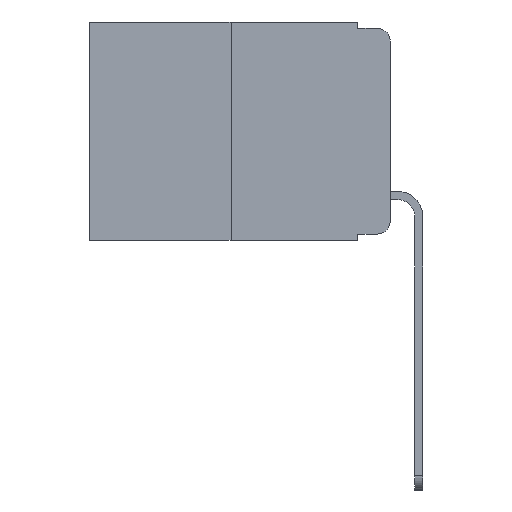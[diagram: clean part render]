
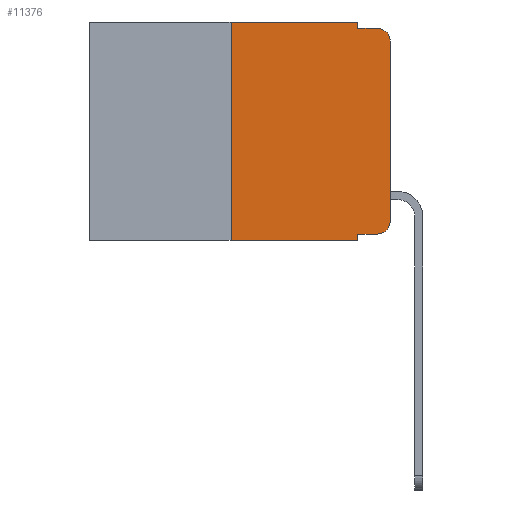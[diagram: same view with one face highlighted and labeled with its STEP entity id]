
A CAD part, left-side view. The second image highlights one B-rep face of the part: STEP entity #11376.
In plain terms, the highlighted planar face has unit normal (-1, 0, 0).
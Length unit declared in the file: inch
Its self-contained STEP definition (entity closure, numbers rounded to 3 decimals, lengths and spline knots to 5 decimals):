
#78 = VERTEX_POINT ( 'NONE', #9142 ) ;
#319 = VECTOR ( 'NONE', #1893, 39.37008 ) ;
#492 = LINE ( 'NONE', #1943, #319 ) ;
#668 = LINE ( 'NONE', #11216, #2247 ) ;
#675 = VECTOR ( 'NONE', #11264, 39.37008 ) ;
#968 = PLANE ( 'NONE',  #13444 ) ;
#1014 = DIRECTION ( 'NONE',  ( 1., 0., 0. ) ) ;
#1072 = DIRECTION ( 'NONE',  ( -1., 0., 0. ) ) ;
#1408 = VECTOR ( 'NONE', #3581, 39.37008 ) ;
#1508 = VECTOR ( 'NONE', #7893, 39.37008 ) ;
#1582 = EDGE_CURVE ( 'NONE', #3085, #9152, #4040, .T. ) ;
#1893 = DIRECTION ( 'NONE',  ( 0., -1., 0. ) ) ;
#1917 = AXIS2_PLACEMENT_3D ( 'NONE', #4322, #4279, #14426 ) ;
#1943 = CARTESIAN_POINT ( 'NONE',  ( 0., 0.051, -0.333 ) ) ;
#2247 = VECTOR ( 'NONE', #13514, 39.37008 ) ;
#2286 = ORIENTED_EDGE ( 'NONE', *, *, #2820, .F. ) ;
#2370 = CARTESIAN_POINT ( 'NONE',  ( 0., 0., 0. ) ) ;
#2820 = EDGE_CURVE ( 'NONE', #6180, #4557, #9934, .T. ) ;
#2931 = EDGE_CURVE ( 'NONE', #7066, #6180, #6783, .T. ) ;
#3085 = VERTEX_POINT ( 'NONE', #10618 ) ;
#3165 = CARTESIAN_POINT ( 'NONE',  ( 0., 0.051, -0.343 ) ) ;
#3506 = CARTESIAN_POINT ( 'NONE',  ( 0., 0.051, 0. ) ) ;
#3535 = CARTESIAN_POINT ( 'NONE',  ( 0., 0.051, -0.01 ) ) ;
#3581 = DIRECTION ( 'NONE',  ( 0., -1., 0. ) ) ;
#3651 = VERTEX_POINT ( 'NONE', #8904 ) ;
#3710 = EDGE_CURVE ( 'NONE', #7066, #8391, #3791, .T. ) ;
#3791 = LINE ( 'NONE', #4683, #1508 ) ;
#4040 = LINE ( 'NONE', #3535, #1408 ) ;
#4217 = ORIENTED_EDGE ( 'NONE', *, *, #2931, .F. ) ;
#4246 = LINE ( 'NONE', #3506, #10911 ) ;
#4269 = ORIENTED_EDGE ( 'NONE', *, *, #10042, .T. ) ;
#4279 = DIRECTION ( 'NONE',  ( -1., 0., 0. ) ) ;
#4322 = CARTESIAN_POINT ( 'NONE',  ( 0., 0.02, -0.03 ) ) ;
#4323 = CARTESIAN_POINT ( 'NONE',  ( 0., 0.051, 0. ) ) ;
#4557 = VERTEX_POINT ( 'NONE', #4323 ) ;
#4683 = CARTESIAN_POINT ( 'NONE',  ( 0., 0.473, -0.343 ) ) ;
#4719 = VECTOR ( 'NONE', #11214, 39.37008 ) ;
#5251 = CIRCLE ( 'NONE', #7163, 0.02 ) ;
#5389 = VERTEX_POINT ( 'NONE', #7640 ) ;
#5499 = DIRECTION ( 'NONE',  ( 0., 0., -1. ) ) ;
#5584 = CARTESIAN_POINT ( 'NONE',  ( 0., 0.25, 0. ) ) ;
#5716 = CIRCLE ( 'NONE', #1917, 0.02 ) ;
#5769 = LINE ( 'NONE', #2370, #4719 ) ;
#5912 = VECTOR ( 'NONE', #14518, 39.37008 ) ;
#6067 = EDGE_CURVE ( 'NONE', #5389, #3651, #5769, .T. ) ;
#6147 = ORIENTED_EDGE ( 'NONE', *, *, #6067, .T. ) ;
#6180 = VERTEX_POINT ( 'NONE', #13803 ) ;
#6581 = EDGE_CURVE ( 'NONE', #78, #5389, #5251, .T. ) ;
#6583 = CARTESIAN_POINT ( 'NONE',  ( 0., 0.473, 0. ) ) ;
#6783 = LINE ( 'NONE', #5584, #675 ) ;
#7066 = VERTEX_POINT ( 'NONE', #7863 ) ;
#7163 = AXIS2_PLACEMENT_3D ( 'NONE', #7831, #1072, #10055 ) ;
#7392 = ORIENTED_EDGE ( 'NONE', *, *, #6581, .T. ) ;
#7640 = CARTESIAN_POINT ( 'NONE',  ( 0., 0., -0.313 ) ) ;
#7831 = CARTESIAN_POINT ( 'NONE',  ( 0., 0.02, -0.313 ) ) ;
#7863 = CARTESIAN_POINT ( 'NONE',  ( 0., 0.25, -0.343 ) ) ;
#7893 = DIRECTION ( 'NONE',  ( 0., -1., 0. ) ) ;
#7967 = ORIENTED_EDGE ( 'NONE', *, *, #11808, .T. ) ;
#8049 = CARTESIAN_POINT ( 'NONE',  ( 0., 0.02, -0.01 ) ) ;
#8322 = DIRECTION ( 'NONE',  ( 0., 0., -1. ) ) ;
#8391 = VERTEX_POINT ( 'NONE', #3165 ) ;
#8743 = FACE_OUTER_BOUND ( 'NONE', #14047, .T. ) ;
#8785 = VERTEX_POINT ( 'NONE', #13934 ) ;
#8904 = CARTESIAN_POINT ( 'NONE',  ( 0., 0., -0.03 ) ) ;
#9142 = CARTESIAN_POINT ( 'NONE',  ( 0., 0.02, -0.333 ) ) ;
#9152 = VERTEX_POINT ( 'NONE', #8049 ) ;
#9666 = EDGE_CURVE ( 'NONE', #4557, #3085, #4246, .T. ) ;
#9934 = LINE ( 'NONE', #12184, #5912 ) ;
#10042 = EDGE_CURVE ( 'NONE', #3651, #9152, #5716, .T. ) ;
#10055 = DIRECTION ( 'NONE',  ( 0., 0., -1. ) ) ;
#10107 = ORIENTED_EDGE ( 'NONE', *, *, #1582, .F. ) ;
#10618 = CARTESIAN_POINT ( 'NONE',  ( 0., 0.051, -0.01 ) ) ;
#10911 = VECTOR ( 'NONE', #8322, 39.37008 ) ;
#10939 = ORIENTED_EDGE ( 'NONE', *, *, #12084, .F. ) ;
#11060 = ORIENTED_EDGE ( 'NONE', *, *, #9666, .F. ) ;
#11214 = DIRECTION ( 'NONE',  ( 0., 0., 1. ) ) ;
#11216 = CARTESIAN_POINT ( 'NONE',  ( 0., 0.051, 0. ) ) ;
#11264 = DIRECTION ( 'NONE',  ( 0., 0., 1. ) ) ;
#11376 = ADVANCED_FACE ( 'NONE', ( #8743 ), #968, .F. ) ;
#11808 = EDGE_CURVE ( 'NONE', #8785, #78, #492, .T. ) ;
#12084 = EDGE_CURVE ( 'NONE', #8785, #8391, #668, .T. ) ;
#12184 = CARTESIAN_POINT ( 'NONE',  ( 0., 0.473, 0. ) ) ;
#13444 = AXIS2_PLACEMENT_3D ( 'NONE', #6583, #1014, #5499 ) ;
#13514 = DIRECTION ( 'NONE',  ( 0., 0., -1. ) ) ;
#13588 = ORIENTED_EDGE ( 'NONE', *, *, #3710, .T. ) ;
#13803 = CARTESIAN_POINT ( 'NONE',  ( 0., 0.25, 0. ) ) ;
#13934 = CARTESIAN_POINT ( 'NONE',  ( 0., 0.051, -0.333 ) ) ;
#14047 = EDGE_LOOP ( 'NONE', ( #6147, #4269, #10107, #11060, #2286, #4217, #13588, #10939, #7967, #7392 ) ) ;
#14426 = DIRECTION ( 'NONE',  ( 0., 0., -1. ) ) ;
#14518 = DIRECTION ( 'NONE',  ( 0., -1., 0. ) ) ;
